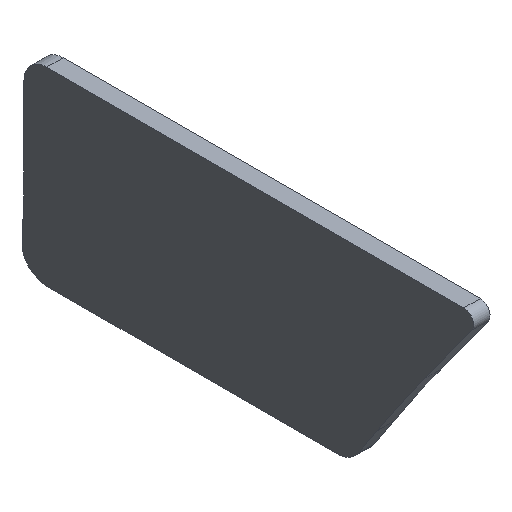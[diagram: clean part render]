
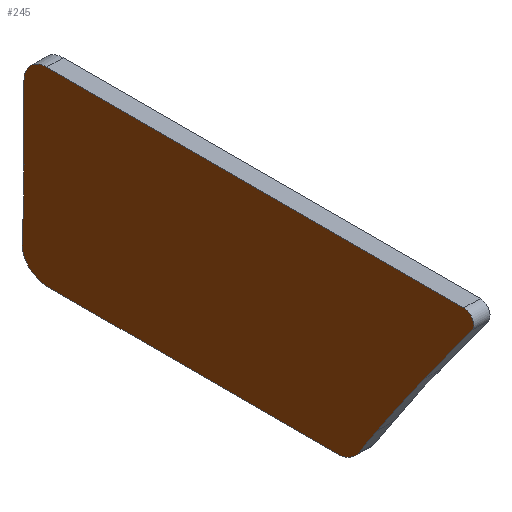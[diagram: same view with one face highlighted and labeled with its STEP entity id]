
A CAD part, isometric view. The second image highlights one B-rep face of the part: STEP entity #245.
In plain terms, the highlighted planar face has unit normal (-1, 0, 0).
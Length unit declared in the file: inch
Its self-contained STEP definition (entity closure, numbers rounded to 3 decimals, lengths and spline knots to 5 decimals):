
#23=FACE_OUTER_BOUND('',#37,.T.);
#37=EDGE_LOOP('',(#167,#168,#169,#170,#171,#172,#173,#174,#175,#176,#177,
#178));
#51=B_SPLINE_CURVE_WITH_KNOTS('',3,(#367,#368,#369,#370,#371,#372,#373),
 .UNSPECIFIED.,.F.,.F.,(4,3,4),(-0.24337,-0.1043,0.),
 .UNSPECIFIED.);
#52=B_SPLINE_CURVE_WITH_KNOTS('',3,(#377,#378,#379,#380,#381,#382,#383,
#384),.UNSPECIFIED.,.F.,.F.,(4,2,2,4),(-0.19113,-0.131,
-0.07087,0.),.UNSPECIFIED.);
#53=B_SPLINE_CURVE_WITH_KNOTS('',3,(#386,#387,#388,#389,#390,#391),
 .UNSPECIFIED.,.F.,.F.,(4,2,4),(-0.26959,-0.1348,0.),
 .UNSPECIFIED.);
#57=ELLIPSE('',#276,0.55083,0.08);
#58=ELLIPSE('',#277,0.07231,0.06261);
#59=ELLIPSE('',#278,0.67725,0.08);
#63=CIRCLE('',#274,0.03);
#64=CIRCLE('',#275,0.07);
#67=LINE('',#353,#87);
#68=LINE('',#357,#88);
#69=LINE('',#361,#89);
#70=LINE('',#375,#90);
#87=VECTOR('',#295,0.3937);
#88=VECTOR('',#298,0.3937);
#89=VECTOR('',#301,0.3937);
#90=VECTOR('',#306,0.3937);
#107=VERTEX_POINT('',#351);
#108=VERTEX_POINT('',#352);
#109=VERTEX_POINT('',#354);
#110=VERTEX_POINT('',#356);
#111=VERTEX_POINT('',#358);
#112=VERTEX_POINT('',#360);
#113=VERTEX_POINT('',#362);
#114=VERTEX_POINT('',#364);
#115=VERTEX_POINT('',#366);
#116=VERTEX_POINT('',#374);
#117=VERTEX_POINT('',#376);
#118=VERTEX_POINT('',#385);
#131=EDGE_CURVE('',#107,#108,#67,.T.);
#132=EDGE_CURVE('',#109,#107,#63,.T.);
#133=EDGE_CURVE('',#110,#109,#68,.T.);
#134=EDGE_CURVE('',#111,#110,#64,.T.);
#135=EDGE_CURVE('',#112,#111,#69,.T.);
#136=EDGE_CURVE('',#113,#112,#57,.T.);
#137=EDGE_CURVE('',#114,#113,#58,.T.);
#138=EDGE_CURVE('',#115,#114,#51,.T.);
#139=EDGE_CURVE('',#116,#115,#70,.T.);
#140=EDGE_CURVE('',#117,#116,#52,.T.);
#141=EDGE_CURVE('',#118,#117,#53,.T.);
#142=EDGE_CURVE('',#108,#118,#59,.T.);
#167=ORIENTED_EDGE('',*,*,#131,.F.);
#168=ORIENTED_EDGE('',*,*,#132,.F.);
#169=ORIENTED_EDGE('',*,*,#133,.F.);
#170=ORIENTED_EDGE('',*,*,#134,.F.);
#171=ORIENTED_EDGE('',*,*,#135,.F.);
#172=ORIENTED_EDGE('',*,*,#136,.F.);
#173=ORIENTED_EDGE('',*,*,#137,.F.);
#174=ORIENTED_EDGE('',*,*,#138,.F.);
#175=ORIENTED_EDGE('',*,*,#139,.F.);
#176=ORIENTED_EDGE('',*,*,#140,.F.);
#177=ORIENTED_EDGE('',*,*,#141,.F.);
#178=ORIENTED_EDGE('',*,*,#142,.F.);
#239=PLANE('',#273);
#245=ADVANCED_FACE('',(#23),#239,.T.);
#273=AXIS2_PLACEMENT_3D('',#350,#293,#294);
#274=AXIS2_PLACEMENT_3D('',#355,#296,#297);
#275=AXIS2_PLACEMENT_3D('',#359,#299,#300);
#276=AXIS2_PLACEMENT_3D('',#363,#302,#303);
#277=AXIS2_PLACEMENT_3D('',#365,#304,#305);
#278=AXIS2_PLACEMENT_3D('',#392,#307,#308);
#293=DIRECTION('center_axis',(-1.,0.,0.));
#294=DIRECTION('ref_axis',(0.,0.,1.));
#295=DIRECTION('',(0.,0.586,-0.81));
#296=DIRECTION('center_axis',(1.,0.,0.));
#297=DIRECTION('ref_axis',(0.,-0.81,-0.586));
#298=DIRECTION('',(0.,-1.,0.));
#299=DIRECTION('center_axis',(1.,0.,0.));
#300=DIRECTION('ref_axis',(0.,0.,1.));
#301=DIRECTION('',(0.,0.,1.));
#302=DIRECTION('center_axis',(-1.,0.,0.));
#303=DIRECTION('ref_axis',(0.,0.,-1.));
#304=DIRECTION('center_axis',(1.,0.,0.));
#305=DIRECTION('ref_axis',(0.,-0.036,0.999));
#306=DIRECTION('',(0.,1.,0.));
#307=DIRECTION('center_axis',(-1.,0.,0.));
#308=DIRECTION('ref_axis',(0.,0.586,-0.81));
#350=CARTESIAN_POINT('Origin',(0.295,-1.65145,1.81519));
#351=CARTESIAN_POINT('',(0.295,-2.33675,2.05759));
#352=CARTESIAN_POINT('',(0.295,-2.19304,1.85882));
#353=CARTESIAN_POINT('',(0.295,-2.16158,1.8153));
#354=CARTESIAN_POINT('',(0.295,-2.31244,2.10516));
#355=CARTESIAN_POINT('Origin',(0.295,-2.31244,2.07516));
#356=CARTESIAN_POINT('',(0.295,-1.03725,2.10516));
#357=CARTESIAN_POINT('',(0.295,-1.34435,2.10516));
#358=CARTESIAN_POINT('',(0.295,-0.96725,2.03516));
#359=CARTESIAN_POINT('Origin',(0.295,-1.03725,2.03516));
#360=CARTESIAN_POINT('',(0.295,-0.96725,1.81195));
#361=CARTESIAN_POINT('',(0.295,-0.96725,1.81357));
#362=CARTESIAN_POINT('',(0.295,-0.96137,1.60463));
#363=CARTESIAN_POINT('Origin',(0.295,-0.88725,1.81195));
#364=CARTESIAN_POINT('',(0.295,-0.96132,1.60387));
#365=CARTESIAN_POINT('Origin',(0.295,-1.02385,1.60045));
#366=CARTESIAN_POINT('',(0.295,-1.03725,1.52521));
#367=CARTESIAN_POINT('Ctrl Pts',(0.295,-1.03725,1.52521));
#368=CARTESIAN_POINT('Ctrl Pts',(0.295,-1.01396,1.52521));
#369=CARTESIAN_POINT('Ctrl Pts',(0.295,-0.9909,1.53654));
#370=CARTESIAN_POINT('Ctrl Pts',(0.295,-0.97672,1.55491));
#371=CARTESIAN_POINT('Ctrl Pts',(0.295,-0.96609,1.56869));
#372=CARTESIAN_POINT('Ctrl Pts',(0.295,-0.96045,1.58643));
#373=CARTESIAN_POINT('Ctrl Pts',(0.295,-0.96132,1.60387));
#374=CARTESIAN_POINT('',(0.295,-1.92605,1.52521));
#375=CARTESIAN_POINT('',(0.295,-1.78875,1.52521));
#376=CARTESIAN_POINT('',(0.295,-1.98976,1.55935));
#377=CARTESIAN_POINT('Ctrl Pts',(0.295,-1.98976,1.55935));
#378=CARTESIAN_POINT('Ctrl Pts',(0.295,-1.98542,1.55276));
#379=CARTESIAN_POINT('Ctrl Pts',(0.295,-1.97998,1.54694));
#380=CARTESIAN_POINT('Ctrl Pts',(0.295,-1.9676,1.53716));
#381=CARTESIAN_POINT('Ctrl Pts',(0.295,-1.96065,1.53321));
#382=CARTESIAN_POINT('Ctrl Pts',(0.295,-1.94461,1.52702));
#383=CARTESIAN_POINT('Ctrl Pts',(0.295,-1.93535,1.52521));
#384=CARTESIAN_POINT('Ctrl Pts',(0.295,-1.92605,1.52521));
#385=CARTESIAN_POINT('',(0.295,-2.048,1.64808));
#386=CARTESIAN_POINT('Ctrl Pts',(0.295,-2.048,1.64808));
#387=CARTESIAN_POINT('Ctrl Pts',(0.295,-2.03834,1.63327));
#388=CARTESIAN_POINT('Ctrl Pts',(0.295,-2.02865,1.61847));
#389=CARTESIAN_POINT('Ctrl Pts',(0.295,-2.00923,1.58889));
#390=CARTESIAN_POINT('Ctrl Pts',(0.295,-1.9995,1.57412));
#391=CARTESIAN_POINT('Ctrl Pts',(0.295,-1.98976,1.55935));
#392=CARTESIAN_POINT('Origin',(0.295,-2.25788,1.81195));
